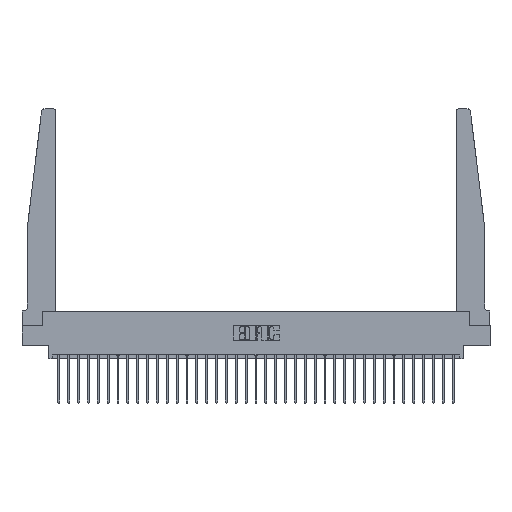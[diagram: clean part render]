
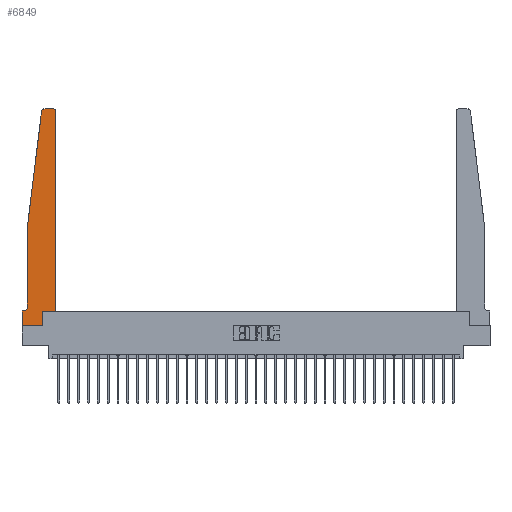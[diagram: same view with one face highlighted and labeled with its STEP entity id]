
A CAD part, top view. The second image highlights one B-rep face of the part: STEP entity #6849.
In plain terms, the highlighted planar face has unit normal (0, 0, 1).
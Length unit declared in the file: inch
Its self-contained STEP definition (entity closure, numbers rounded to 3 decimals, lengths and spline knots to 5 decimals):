
#710 = VERTEX_POINT ( 'NONE', #9390 ) ;
#1088 = VERTEX_POINT ( 'NONE', #27709 ) ;
#1160 = VECTOR ( 'NONE', #10614, 39.37008 ) ;
#1248 = DIRECTION ( 'NONE',  ( -1., 0., 0. ) ) ;
#1459 = LINE ( 'NONE', #8650, #27632 ) ;
#1765 = VERTEX_POINT ( 'NONE', #6303 ) ;
#1875 = CARTESIAN_POINT ( 'NONE',  ( 0.065, 1.25, 0.37 ) ) ;
#1919 = VERTEX_POINT ( 'NONE', #14292 ) ;
#2407 = EDGE_CURVE ( 'NONE', #14442, #4519, #18279, .T. ) ;
#2592 = CARTESIAN_POINT ( 'NONE',  ( 0.395, 2.72, 0.37 ) ) ;
#2598 = EDGE_CURVE ( 'NONE', #28118, #1919, #14454, .T. ) ;
#2627 = ORIENTED_EDGE ( 'NONE', *, *, #6748, .T. ) ;
#4148 = LINE ( 'NONE', #23548, #22246 ) ;
#4437 = AXIS2_PLACEMENT_3D ( 'NONE', #2592, #19804, #5086 ) ;
#4519 = VERTEX_POINT ( 'NONE', #16387 ) ;
#4542 = DIRECTION ( 'NONE',  ( 1., 0., 0. ) ) ;
#5086 = DIRECTION ( 'NONE',  ( 1., 0., 0. ) ) ;
#5964 = VECTOR ( 'NONE', #23253, 39.37008 ) ;
#6138 = EDGE_CURVE ( 'NONE', #4519, #25461, #1459, .T. ) ;
#6303 = CARTESIAN_POINT ( 'NONE',  ( 0.24675, 2.72367, 0.37 ) ) ;
#6748 = EDGE_CURVE ( 'NONE', #1765, #8862, #4148, .T. ) ;
#6849 = ADVANCED_FACE ( 'NONE', ( #26410 ), #31459, .T. ) ;
#7119 = VECTOR ( 'NONE', #17367, 39.37008 ) ;
#7742 = DIRECTION ( 'NONE',  ( 0., 0., 1. ) ) ;
#7891 = LINE ( 'NONE', #27215, #7119 ) ;
#7982 = CARTESIAN_POINT ( 'NONE',  ( 0.2605, 0.18, 0.37 ) ) ;
#8440 = ORIENTED_EDGE ( 'NONE', *, *, #12831, .T. ) ;
#8480 = AXIS2_PLACEMENT_3D ( 'NONE', #30667, #16009, #1248 ) ;
#8650 = CARTESIAN_POINT ( 'NONE',  ( 0.425, 0.18, 0.37 ) ) ;
#8862 = VERTEX_POINT ( 'NONE', #1875 ) ;
#9173 = VECTOR ( 'NONE', #9364, 39.37008 ) ;
#9213 = ORIENTED_EDGE ( 'NONE', *, *, #23634, .T. ) ;
#9364 = DIRECTION ( 'NONE',  ( 1., 0., 0. ) ) ;
#9390 = CARTESIAN_POINT ( 'NONE',  ( 0.015, 0.1875, 0.37 ) ) ;
#9848 = EDGE_CURVE ( 'NONE', #23430, #14442, #20818, .T. ) ;
#10444 = LINE ( 'NONE', #10931, #29969 ) ;
#10614 = DIRECTION ( 'NONE',  ( 0., 1., 0. ) ) ;
#10931 = CARTESIAN_POINT ( 'NONE',  ( 0.065, 0.1875, 0.37 ) ) ;
#11887 = CARTESIAN_POINT ( 'NONE',  ( 0., 0.1875, 0.37 ) ) ;
#11997 = ORIENTED_EDGE ( 'NONE', *, *, #17721, .T. ) ;
#12518 = CIRCLE ( 'NONE', #26616, 0.03 ) ;
#12831 = EDGE_CURVE ( 'NONE', #26663, #710, #13042, .T. ) ;
#13042 = CIRCLE ( 'NONE', #8480, 0.05 ) ;
#13098 = CARTESIAN_POINT ( 'NONE',  ( 0.2605, 0.18, 0.37 ) ) ;
#13417 = CARTESIAN_POINT ( 'NONE',  ( 0.425, 0.18, 0.37 ) ) ;
#13488 = ORIENTED_EDGE ( 'NONE', *, *, #16687, .T. ) ;
#13778 = CARTESIAN_POINT ( 'NONE',  ( 0.27653, 2.75, 0.37 ) ) ;
#13813 = DIRECTION ( 'NONE',  ( -0.122, -0.992, 0. ) ) ;
#14292 = CARTESIAN_POINT ( 'NONE',  ( 0., 0., 0.37 ) ) ;
#14442 = VERTEX_POINT ( 'NONE', #7982 ) ;
#14454 = LINE ( 'NONE', #26326, #31673 ) ;
#14666 = ORIENTED_EDGE ( 'NONE', *, *, #9848, .T. ) ;
#15295 = EDGE_CURVE ( 'NONE', #1088, #30870, #18336, .T. ) ;
#15712 = LINE ( 'NONE', #24068, #9173 ) ;
#16009 = DIRECTION ( 'NONE',  ( 0., 0., -1. ) ) ;
#16387 = CARTESIAN_POINT ( 'NONE',  ( 0.425, 0.18, 0.37 ) ) ;
#16687 = EDGE_CURVE ( 'NONE', #30870, #1765, #12518, .T. ) ;
#16808 = AXIS2_PLACEMENT_3D ( 'NONE', #11887, #19259, #4542 ) ;
#16830 = DIRECTION ( 'NONE',  ( -1., 0., 0. ) ) ;
#17367 = DIRECTION ( 'NONE',  ( 0., -1., 0. ) ) ;
#17721 = EDGE_CURVE ( 'NONE', #25461, #1088, #30425, .T. ) ;
#17932 = CARTESIAN_POINT ( 'NONE',  ( 0.2605, 0., 0.37 ) ) ;
#18279 = LINE ( 'NONE', #13417, #5964 ) ;
#18336 = LINE ( 'NONE', #29023, #24094 ) ;
#19259 = DIRECTION ( 'NONE',  ( 0., 0., 1. ) ) ;
#19804 = DIRECTION ( 'NONE',  ( 0., 0., 1. ) ) ;
#20185 = EDGE_CURVE ( 'NONE', #1919, #23430, #15712, .T. ) ;
#20377 = CARTESIAN_POINT ( 'NONE',  ( 0., 0.1875, 0.37 ) ) ;
#20818 = LINE ( 'NONE', #13098, #1160 ) ;
#22246 = VECTOR ( 'NONE', #13813, 39.37008 ) ;
#22252 = ORIENTED_EDGE ( 'NONE', *, *, #15295, .T. ) ;
#22460 = CARTESIAN_POINT ( 'NONE',  ( 0.27653, 2.72, 0.37 ) ) ;
#23131 = DIRECTION ( 'NONE',  ( -1., 0., 0. ) ) ;
#23253 = DIRECTION ( 'NONE',  ( 1., 0., 0. ) ) ;
#23368 = DIRECTION ( 'NONE',  ( 0., 1., 0. ) ) ;
#23430 = VERTEX_POINT ( 'NONE', #17932 ) ;
#23548 = CARTESIAN_POINT ( 'NONE',  ( 0.065, 1.25, 0.37 ) ) ;
#23634 = EDGE_CURVE ( 'NONE', #710, #28118, #10444, .T. ) ;
#24068 = CARTESIAN_POINT ( 'NONE',  ( 0., 0., 0.37 ) ) ;
#24094 = VECTOR ( 'NONE', #16830, 39.37008 ) ;
#24250 = ORIENTED_EDGE ( 'NONE', *, *, #6138, .T. ) ;
#24572 = ORIENTED_EDGE ( 'NONE', *, *, #29881, .T. ) ;
#24914 = DIRECTION ( 'NONE',  ( 1., 0., 0. ) ) ;
#24946 = EDGE_LOOP ( 'NONE', ( #22252, #13488, #2627, #24572, #8440, #9213, #31103, #25384, #14666, #27689, #24250, #11997 ) ) ;
#25384 = ORIENTED_EDGE ( 'NONE', *, *, #20185, .T. ) ;
#25461 = VERTEX_POINT ( 'NONE', #29891 ) ;
#26326 = CARTESIAN_POINT ( 'NONE',  ( 0., 0., 0.37 ) ) ;
#26410 = FACE_OUTER_BOUND ( 'NONE', #24946, .T. ) ;
#26616 = AXIS2_PLACEMENT_3D ( 'NONE', #22460, #7742, #24914 ) ;
#26663 = VERTEX_POINT ( 'NONE', #31797 ) ;
#27215 = CARTESIAN_POINT ( 'NONE',  ( 0.065, 1.25, 0.37 ) ) ;
#27632 = VECTOR ( 'NONE', #23368, 39.37008 ) ;
#27689 = ORIENTED_EDGE ( 'NONE', *, *, #2407, .T. ) ;
#27709 = CARTESIAN_POINT ( 'NONE',  ( 0.395, 2.75, 0.37 ) ) ;
#28118 = VERTEX_POINT ( 'NONE', #20377 ) ;
#28786 = DIRECTION ( 'NONE',  ( 0., -1., 0. ) ) ;
#29023 = CARTESIAN_POINT ( 'NONE',  ( 0.25, 2.75, 0.37 ) ) ;
#29881 = EDGE_CURVE ( 'NONE', #8862, #26663, #7891, .T. ) ;
#29891 = CARTESIAN_POINT ( 'NONE',  ( 0.425, 2.72, 0.37 ) ) ;
#29969 = VECTOR ( 'NONE', #23131, 39.37008 ) ;
#30425 = CIRCLE ( 'NONE', #4437, 0.03 ) ;
#30667 = CARTESIAN_POINT ( 'NONE',  ( 0.015, 0.2375, 0.37 ) ) ;
#30870 = VERTEX_POINT ( 'NONE', #13778 ) ;
#31103 = ORIENTED_EDGE ( 'NONE', *, *, #2598, .T. ) ;
#31459 = PLANE ( 'NONE',  #16808 ) ;
#31673 = VECTOR ( 'NONE', #28786, 39.37008 ) ;
#31797 = CARTESIAN_POINT ( 'NONE',  ( 0.065, 0.2375, 0.37 ) ) ;
